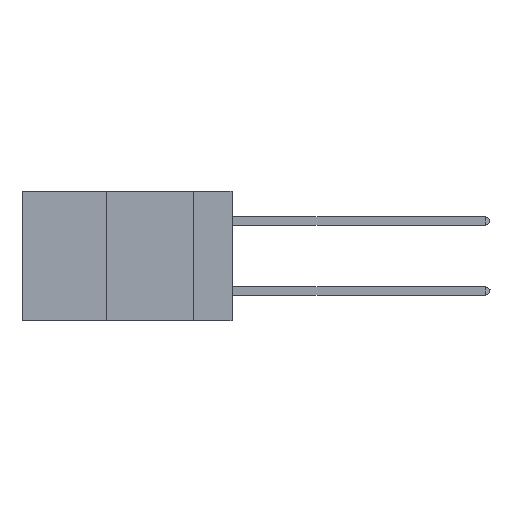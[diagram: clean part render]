
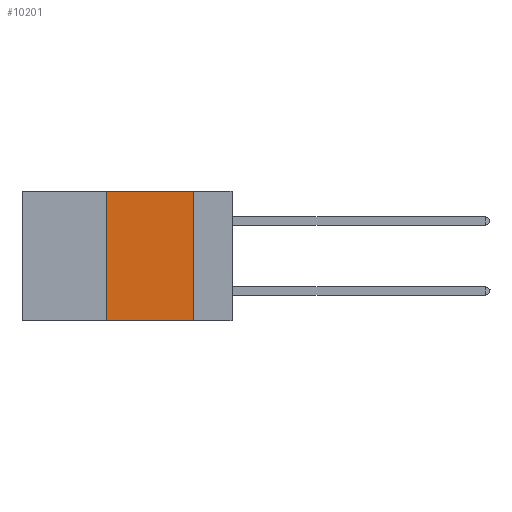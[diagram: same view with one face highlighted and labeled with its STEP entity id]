
A CAD part, left-side view. The second image highlights one B-rep face of the part: STEP entity #10201.
In plain terms, the highlighted planar face has unit normal (-1, 0, 0).
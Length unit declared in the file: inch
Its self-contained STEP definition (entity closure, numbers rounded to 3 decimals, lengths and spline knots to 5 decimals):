
#170 = EDGE_CURVE ( 'NONE', #30104, #30214, #34262, .T. ) ;
#198 = LINE ( 'NONE', #33188, #34800 ) ;
#582 = EDGE_CURVE ( 'NONE', #26020, #30104, #198, .T. ) ;
#1714 = LINE ( 'NONE', #32725, #25948 ) ;
#2117 = DIRECTION ( 'NONE',  ( 0., -1., 0. ) ) ;
#2259 = PLANE ( 'NONE',  #21660 ) ;
#2367 = CARTESIAN_POINT ( 'NONE',  ( 0., 0.11, 0. ) ) ;
#2547 = CARTESIAN_POINT ( 'NONE',  ( 0., 0.6, 0. ) ) ;
#3163 = VERTEX_POINT ( 'NONE', #16987 ) ;
#3284 = DIRECTION ( 'NONE',  ( 0., -1., 0. ) ) ;
#6267 = CARTESIAN_POINT ( 'NONE',  ( 0., 0.11, -0.37 ) ) ;
#8905 = CARTESIAN_POINT ( 'NONE',  ( 0., 0.6, -0.37 ) ) ;
#10201 = ADVANCED_FACE ( 'NONE', ( #30536 ), #2259, .F. ) ;
#12627 = ORIENTED_EDGE ( 'NONE', *, *, #34618, .T. ) ;
#12937 = DIRECTION ( 'NONE',  ( 0., 0., 1. ) ) ;
#13582 = LINE ( 'NONE', #8905, #23362 ) ;
#16987 = CARTESIAN_POINT ( 'NONE',  ( 0., 0.36, -0.37 ) ) ;
#21660 = AXIS2_PLACEMENT_3D ( 'NONE', #2547, #28346, #31572 ) ;
#21834 = VECTOR ( 'NONE', #41955, 39.37008 ) ;
#23362 = VECTOR ( 'NONE', #2117, 39.37008 ) ;
#25948 = VECTOR ( 'NONE', #12937, 39.37008 ) ;
#26020 = VERTEX_POINT ( 'NONE', #35308 ) ;
#27826 = EDGE_CURVE ( 'NONE', #3163, #26020, #1714, .T. ) ;
#28346 = DIRECTION ( 'NONE',  ( 1., 0., 0. ) ) ;
#28616 = CARTESIAN_POINT ( 'NONE',  ( 0., 0.11, 0. ) ) ;
#30104 = VERTEX_POINT ( 'NONE', #2367 ) ;
#30214 = VERTEX_POINT ( 'NONE', #6267 ) ;
#30536 = FACE_OUTER_BOUND ( 'NONE', #38930, .T. ) ;
#31572 = DIRECTION ( 'NONE',  ( 0., 0., -1. ) ) ;
#32725 = CARTESIAN_POINT ( 'NONE',  ( 0., 0.36, 0. ) ) ;
#33188 = CARTESIAN_POINT ( 'NONE',  ( 0., 0.6, 0. ) ) ;
#34262 = LINE ( 'NONE', #28616, #21834 ) ;
#34618 = EDGE_CURVE ( 'NONE', #3163, #30214, #13582, .T. ) ;
#34800 = VECTOR ( 'NONE', #3284, 39.37008 ) ;
#35308 = CARTESIAN_POINT ( 'NONE',  ( 0., 0.36, 0. ) ) ;
#36555 = ORIENTED_EDGE ( 'NONE', *, *, #170, .F. ) ;
#38930 = EDGE_LOOP ( 'NONE', ( #36555, #41500, #42235, #12627 ) ) ;
#41500 = ORIENTED_EDGE ( 'NONE', *, *, #582, .F. ) ;
#41955 = DIRECTION ( 'NONE',  ( 0., 0., -1. ) ) ;
#42235 = ORIENTED_EDGE ( 'NONE', *, *, #27826, .F. ) ;
